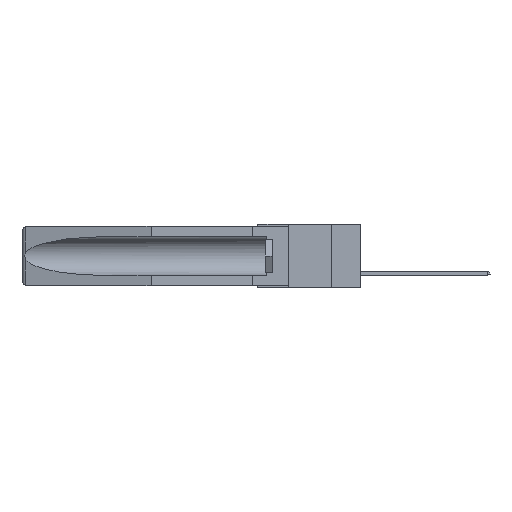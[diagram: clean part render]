
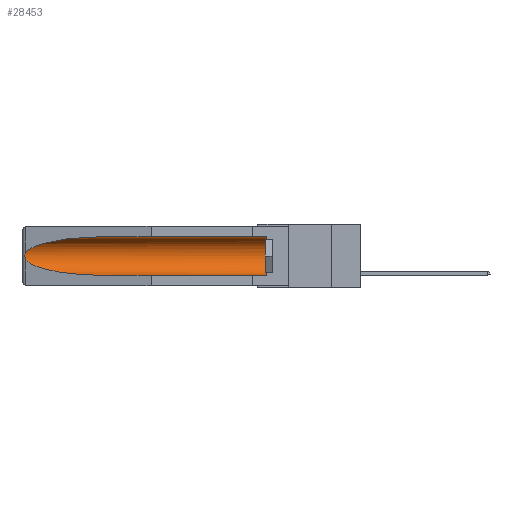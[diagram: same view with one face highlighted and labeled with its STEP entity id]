
A CAD part, left-side view. The second image highlights one B-rep face of the part: STEP entity #28453.
In plain terms, the highlighted cylindrical face has radius 2.857 mm (diameter 5.715 mm), a partial arc.
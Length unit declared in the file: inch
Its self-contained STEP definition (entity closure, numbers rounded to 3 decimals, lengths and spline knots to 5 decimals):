
#137 = EDGE_CURVE ( 'NONE', #21963, #31115, #28569, .T. ) ;
#786 = VERTEX_POINT ( 'NONE', #28262 ) ;
#1246 = LINE ( 'NONE', #15762, #30768 ) ;
#1751 = FACE_OUTER_BOUND ( 'NONE', #27007, .T. ) ;
#2577 = CARTESIAN_POINT ( 'NONE',  ( 0.26537, 1.52718, -0.14972 ) ) ;
#2791 = CARTESIAN_POINT ( 'NONE',  ( 0.21114, 1.30732, -0.059 ) ) ;
#2931 = VERTEX_POINT ( 'NONE', #26907 ) ;
#3078 = CARTESIAN_POINT ( 'NONE',  ( 0.26597, 1.52961, -0.15275 ) ) ;
#3335 = ORIENTED_EDGE ( 'NONE', *, *, #9582, .T. ) ;
#4474 = CARTESIAN_POINT ( 'NONE',  ( 0.155, 1.07973, -0.284 ) ) ;
#4920 = DIRECTION ( 'NONE',  ( 0., 0., 1. ) ) ;
#5077 = AXIS2_PLACEMENT_3D ( 'NONE', #17276, #14077, #4920 ) ;
#5230 = LINE ( 'NONE', #18424, #14761 ) ;
#5508 = CARTESIAN_POINT ( 'NONE',  ( 0.26597, 1.5296, -0.19026 ) ) ;
#8056 = ORIENTED_EDGE ( 'NONE', *, *, #19429, .F. ) ;
#8254 = CARTESIAN_POINT ( 'NONE',  ( 0.2675, 1.53308, -0.17534 ) ) ;
#8715 = DIRECTION ( 'NONE',  ( 0., 1., 0. ) ) ;
#9381 = CARTESIAN_POINT ( 'NONE',  ( 0.155, 0.126, -0.059 ) ) ;
#9491 = CARTESIAN_POINT ( 'NONE',  ( 0.155, 0.126, -0.284 ) ) ;
#9582 = EDGE_CURVE ( 'NONE', #25286, #28284, #24058, .T. ) ;
#9585 = EDGE_CURVE ( 'NONE', #786, #2931, #28169, .T. ) ;
#10741 = CARTESIAN_POINT ( 'NONE',  ( 0.2673, 1.53269, -0.17917 ) ) ;
#11543 = ORIENTED_EDGE ( 'NONE', *, *, #137, .T. ) ;
#12563 = DIRECTION ( 'NONE',  ( 0., 1., 0. ) ) ;
#12956 = CARTESIAN_POINT ( 'NONE',  ( 0.26537, 1.52718, -0.14972 ) ) ;
#13806 = CARTESIAN_POINT ( 'NONE',  ( 0.26537, 1.52718, -0.19328 ) ) ;
#14077 = DIRECTION ( 'NONE',  ( 0., -1., 0. ) ) ;
#14761 = VECTOR ( 'NONE', #8715, 39.37008 ) ;
#14917 = CARTESIAN_POINT ( 'NONE',  ( 0.155, -0.30754, -0.1715 ) ) ;
#15762 = CARTESIAN_POINT ( 'NONE',  ( 0.155, -0.30754, -0.059 ) ) ;
#16116 = ORIENTED_EDGE ( 'NONE', *, *, #20207, .T. ) ;
#16363 = CARTESIAN_POINT ( 'NONE',  ( 0.155, 1.07973, -0.284 ) ) ;
#17176 = CARTESIAN_POINT ( 'NONE',  ( 0.155, 1.07973, -0.059 ) ) ;
#17276 = CARTESIAN_POINT ( 'NONE',  ( 0.155, 0.126, -0.1715 ) ) ;
#17778 = ORIENTED_EDGE ( 'NONE', *, *, #24373, .T. ) ;
#18424 = CARTESIAN_POINT ( 'NONE',  ( 0.155, -0.30754, -0.284 ) ) ;
#19045 = CARTESIAN_POINT ( 'NONE',  ( 0.21114, 1.30732, -0.284 ) ) ;
#19251 = CARTESIAN_POINT ( 'NONE',  ( 0.26537, 1.52718, -0.19328 ) ) ;
#19429 = EDGE_CURVE ( 'NONE', #25286, #31115, #5230, .T. ) ;
#19511 = DIRECTION ( 'NONE',  ( 0., 0., 1. ) ) ;
#20121 = CARTESIAN_POINT ( 'NONE',  ( 0.26655, 1.53094, -0.18657 ) ) ;
#20207 = EDGE_CURVE ( 'NONE', #28284, #786, #1246, .T. ) ;
#21523 = CARTESIAN_POINT ( 'NONE',  ( 0.25451, 1.48313, -0.24835 ) ) ;
#21963 = VERTEX_POINT ( 'NONE', #27057 ) ;
#22931 = CARTESIAN_POINT ( 'NONE',  ( 0.2673, 1.5327, -0.16383 ) ) ;
#22949 = AXIS2_PLACEMENT_3D ( 'NONE', #14917, #12563, #19511 ) ;
#24058 = CIRCLE ( 'NONE', #5077, 0.1125 ) ;
#24373 = EDGE_CURVE ( 'NONE', #2931, #21963, #26197, .T. ) ;
#25286 = VERTEX_POINT ( 'NONE', #9491 ) ;
#25297 = CARTESIAN_POINT ( 'NONE',  ( 0.2675, 1.53308, -0.16763 ) ) ;
#26197 = B_SPLINE_CURVE_WITH_KNOTS ( 'NONE', 3,
 ( #12956, #3078, #30181, #22931, #25297, #8254, #10741, #20121, #5508, #13806 ),
 .UNSPECIFIED., .F., .F.,
 ( 4, 2, 2, 2, 4 ),
 ( 0., 0.00029, 0.00058, 0.00087, 0.00117 ),
 .UNSPECIFIED. ) ;
#26907 = CARTESIAN_POINT ( 'NONE',  ( 0.26537, 1.52718, -0.14972 ) ) ;
#27007 = EDGE_LOOP ( 'NONE', ( #29820, #17778, #11543, #8056, #3335, #16116 ) ) ;
#27017 = CYLINDRICAL_SURFACE ( 'NONE', #22949, 0.1125 ) ;
#27057 = CARTESIAN_POINT ( 'NONE',  ( 0.26537, 1.52718, -0.19328 ) ) ;
#28024 = DIRECTION ( 'NONE',  ( 0., 1., 0. ) ) ;
#28169 =( BOUNDED_CURVE ( )  B_SPLINE_CURVE ( 3, ( #17176, #2791, #29584, #2577 ),
 .UNSPECIFIED., .F., .F. ) 
 B_SPLINE_CURVE_WITH_KNOTS ( ( 4, 4 ),
 ( 4.71239, 6.08839 ),
 .UNSPECIFIED. ) 
 CURVE ( )  GEOMETRIC_REPRESENTATION_ITEM ( )  RATIONAL_B_SPLINE_CURVE ( ( 1., 0.848, 0.848, 1. ) ) 
 REPRESENTATION_ITEM ( '' )  );
#28262 = CARTESIAN_POINT ( 'NONE',  ( 0.155, 1.07973, -0.059 ) ) ;
#28284 = VERTEX_POINT ( 'NONE', #9381 ) ;
#28453 = ADVANCED_FACE ( 'NONE', ( #1751 ), #27017, .F. ) ;
#28569 =( BOUNDED_CURVE ( )  B_SPLINE_CURVE ( 3, ( #19251, #21523, #19045, #4474 ),
 .UNSPECIFIED., .F., .F. ) 
 B_SPLINE_CURVE_WITH_KNOTS ( ( 4, 4 ),
 ( 0.1948, 1.5708 ),
 .UNSPECIFIED. ) 
 CURVE ( )  GEOMETRIC_REPRESENTATION_ITEM ( )  RATIONAL_B_SPLINE_CURVE ( ( 1., 0.848, 0.848, 1. ) ) 
 REPRESENTATION_ITEM ( '' )  );
#29584 = CARTESIAN_POINT ( 'NONE',  ( 0.25451, 1.48313, -0.09465 ) ) ;
#29820 = ORIENTED_EDGE ( 'NONE', *, *, #9585, .T. ) ;
#30181 = CARTESIAN_POINT ( 'NONE',  ( 0.26654, 1.53092, -0.15636 ) ) ;
#30768 = VECTOR ( 'NONE', #28024, 39.37008 ) ;
#31115 = VERTEX_POINT ( 'NONE', #16363 ) ;
